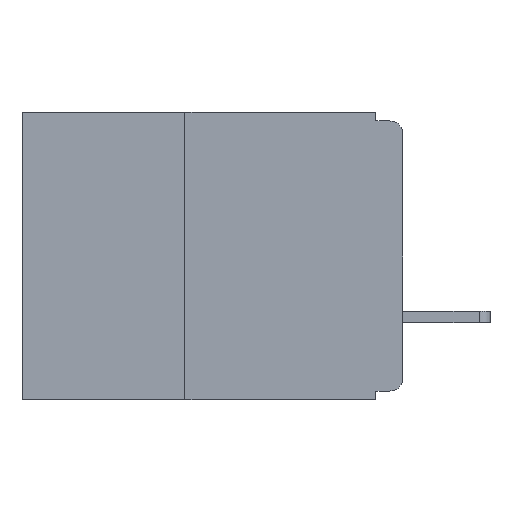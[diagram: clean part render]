
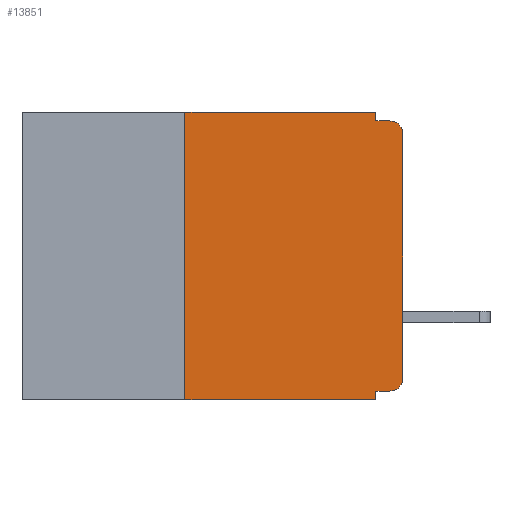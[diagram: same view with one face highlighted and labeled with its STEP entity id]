
A CAD part, left-side view. The second image highlights one B-rep face of the part: STEP entity #13851.
In plain terms, the highlighted planar face has unit normal (-1, 0, 0).
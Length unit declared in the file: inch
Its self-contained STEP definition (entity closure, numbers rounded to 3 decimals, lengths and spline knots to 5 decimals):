
#236 = CIRCLE ( 'NONE', #13794, 0.015 ) ;
#931 = EDGE_CURVE ( 'NONE', #6489, #3420, #7613, .T. ) ;
#1076 = VECTOR ( 'NONE', #17019, 39.37008 ) ;
#1198 = VERTEX_POINT ( 'NONE', #16589 ) ;
#1199 = ORIENTED_EDGE ( 'NONE', *, *, #8540, .F. ) ;
#1265 = ORIENTED_EDGE ( 'NONE', *, *, #11368, .T. ) ;
#1776 = LINE ( 'NONE', #10349, #8502 ) ;
#1939 = CARTESIAN_POINT ( 'NONE',  ( 0., 0.031, -0.32 ) ) ;
#2230 = DIRECTION ( 'NONE',  ( 1., 0., 0. ) ) ;
#2257 = ORIENTED_EDGE ( 'NONE', *, *, #5823, .F. ) ;
#2461 = CARTESIAN_POINT ( 'NONE',  ( 0., 0.25, -0.33 ) ) ;
#2841 = VERTEX_POINT ( 'NONE', #16107 ) ;
#3072 = ORIENTED_EDGE ( 'NONE', *, *, #11194, .T. ) ;
#3173 = CARTESIAN_POINT ( 'NONE',  ( 0., 0.031, 0. ) ) ;
#3230 = DIRECTION ( 'NONE',  ( -1., 0., 0. ) ) ;
#3371 = EDGE_CURVE ( 'NONE', #12981, #3420, #1776, .T. ) ;
#3420 = VERTEX_POINT ( 'NONE', #9836 ) ;
#3835 = ORIENTED_EDGE ( 'NONE', *, *, #8980, .F. ) ;
#3908 = FACE_OUTER_BOUND ( 'NONE', #9179, .T. ) ;
#4218 = ORIENTED_EDGE ( 'NONE', *, *, #12426, .F. ) ;
#4885 = PLANE ( 'NONE',  #7596 ) ;
#5056 = CARTESIAN_POINT ( 'NONE',  ( 0., 0.031, 0. ) ) ;
#5523 = CARTESIAN_POINT ( 'NONE',  ( 0., 0.25, 0. ) ) ;
#5823 = EDGE_CURVE ( 'NONE', #13924, #2841, #9790, .T. ) ;
#5826 = CARTESIAN_POINT ( 'NONE',  ( 0., 0.015, -0.025 ) ) ;
#5854 = VERTEX_POINT ( 'NONE', #9881 ) ;
#6044 = DIRECTION ( 'NONE',  ( 0., -1., 0. ) ) ;
#6489 = VERTEX_POINT ( 'NONE', #1939 ) ;
#6513 = DIRECTION ( 'NONE',  ( 0., 0., 1. ) ) ;
#6645 = CARTESIAN_POINT ( 'NONE',  ( 0., 0.437, 0. ) ) ;
#6756 = ORIENTED_EDGE ( 'NONE', *, *, #3371, .T. ) ;
#6946 = VECTOR ( 'NONE', #14624, 39.37008 ) ;
#6959 = CIRCLE ( 'NONE', #10928, 0.015 ) ;
#7168 = DIRECTION ( 'NONE',  ( 0., 0., -1. ) ) ;
#7248 = VECTOR ( 'NONE', #6513, 39.37008 ) ;
#7596 = AXIS2_PLACEMENT_3D ( 'NONE', #10202, #2230, #11515 ) ;
#7613 = LINE ( 'NONE', #12077, #14549 ) ;
#7879 = LINE ( 'NONE', #6645, #1076 ) ;
#7890 = CARTESIAN_POINT ( 'NONE',  ( 0., 0.25, -0.33 ) ) ;
#7912 = CARTESIAN_POINT ( 'NONE',  ( 0., 0., -0.025 ) ) ;
#8424 = VECTOR ( 'NONE', #6044, 39.37008 ) ;
#8502 = VECTOR ( 'NONE', #10437, 39.37008 ) ;
#8540 = EDGE_CURVE ( 'NONE', #12981, #14148, #14190, .T. ) ;
#8609 = ORIENTED_EDGE ( 'NONE', *, *, #16156, .F. ) ;
#8980 = EDGE_CURVE ( 'NONE', #2841, #5854, #11108, .T. ) ;
#9179 = EDGE_LOOP ( 'NONE', ( #3072, #12849, #3835, #2257, #4218, #1199, #6756, #11718, #8609, #1265 ) ) ;
#9503 = CARTESIAN_POINT ( 'NONE',  ( 0., 0., -0.32 ) ) ;
#9790 = LINE ( 'NONE', #3173, #15895 ) ;
#9827 = DIRECTION ( 'NONE',  ( 0., 0., -1. ) ) ;
#9836 = CARTESIAN_POINT ( 'NONE',  ( 0., 0.031, -0.33 ) ) ;
#9851 = VERTEX_POINT ( 'NONE', #7912 ) ;
#9881 = CARTESIAN_POINT ( 'NONE',  ( 0., 0.015, -0.01 ) ) ;
#10202 = CARTESIAN_POINT ( 'NONE',  ( 0., 0.437, 0. ) ) ;
#10349 = CARTESIAN_POINT ( 'NONE',  ( 0., 0.437, -0.33 ) ) ;
#10437 = DIRECTION ( 'NONE',  ( 0., -1., 0. ) ) ;
#10714 = EDGE_CURVE ( 'NONE', #9851, #5854, #6959, .T. ) ;
#10816 = DIRECTION ( 'NONE',  ( 0., 1., 0. ) ) ;
#10819 = LINE ( 'NONE', #13336, #6946 ) ;
#10928 = AXIS2_PLACEMENT_3D ( 'NONE', #5826, #14982, #7168 ) ;
#11108 = LINE ( 'NONE', #12628, #8424 ) ;
#11146 = CARTESIAN_POINT ( 'NONE',  ( 0., 0.015, -0.305 ) ) ;
#11194 = EDGE_CURVE ( 'NONE', #13032, #9851, #10819, .T. ) ;
#11368 = EDGE_CURVE ( 'NONE', #1198, #13032, #236, .T. ) ;
#11515 = DIRECTION ( 'NONE',  ( 0., 0., -1. ) ) ;
#11718 = ORIENTED_EDGE ( 'NONE', *, *, #931, .F. ) ;
#11808 = DIRECTION ( 'NONE',  ( 0., 0., -1. ) ) ;
#12077 = CARTESIAN_POINT ( 'NONE',  ( 0., 0.031, -0.33 ) ) ;
#12426 = EDGE_CURVE ( 'NONE', #14148, #13924, #7879, .T. ) ;
#12459 = DIRECTION ( 'NONE',  ( 0., 0., -1. ) ) ;
#12628 = CARTESIAN_POINT ( 'NONE',  ( 0., 0., -0.01 ) ) ;
#12849 = ORIENTED_EDGE ( 'NONE', *, *, #10714, .T. ) ;
#12981 = VERTEX_POINT ( 'NONE', #7890 ) ;
#13032 = VERTEX_POINT ( 'NONE', #15808 ) ;
#13336 = CARTESIAN_POINT ( 'NONE',  ( 0., 0., 0. ) ) ;
#13739 = VECTOR ( 'NONE', #10816, 39.37008 ) ;
#13794 = AXIS2_PLACEMENT_3D ( 'NONE', #11146, #3230, #12459 ) ;
#13851 = ADVANCED_FACE ( 'NONE', ( #3908 ), #4885, .F. ) ;
#13924 = VERTEX_POINT ( 'NONE', #5056 ) ;
#14148 = VERTEX_POINT ( 'NONE', #5523 ) ;
#14190 = LINE ( 'NONE', #2461, #7248 ) ;
#14549 = VECTOR ( 'NONE', #11808, 39.37008 ) ;
#14624 = DIRECTION ( 'NONE',  ( 0., 0., 1. ) ) ;
#14982 = DIRECTION ( 'NONE',  ( -1., 0., 0. ) ) ;
#15808 = CARTESIAN_POINT ( 'NONE',  ( 0., 0., -0.305 ) ) ;
#15895 = VECTOR ( 'NONE', #9827, 39.37008 ) ;
#16107 = CARTESIAN_POINT ( 'NONE',  ( 0., 0.031, -0.01 ) ) ;
#16156 = EDGE_CURVE ( 'NONE', #1198, #6489, #17112, .T. ) ;
#16589 = CARTESIAN_POINT ( 'NONE',  ( 0., 0.015, -0.32 ) ) ;
#17019 = DIRECTION ( 'NONE',  ( 0., -1., 0. ) ) ;
#17112 = LINE ( 'NONE', #9503, #13739 ) ;
